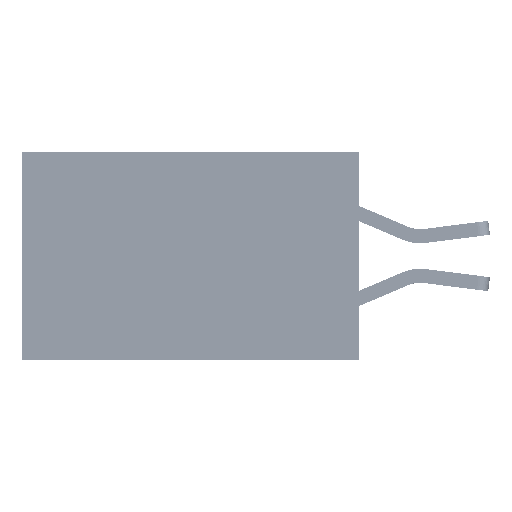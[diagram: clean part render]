
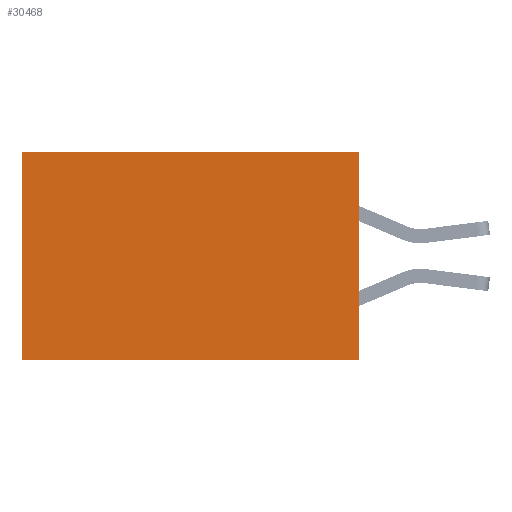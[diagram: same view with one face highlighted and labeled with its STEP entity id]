
A CAD part, left-side view. The second image highlights one B-rep face of the part: STEP entity #30468.
In plain terms, the highlighted planar face has unit normal (-1, 0, 0).
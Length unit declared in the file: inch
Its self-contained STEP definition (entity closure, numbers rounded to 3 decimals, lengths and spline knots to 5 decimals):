
#4207 = LINE ( 'NONE', #34010, #36794 ) ;
#5141 = ORIENTED_EDGE ( 'NONE', *, *, #14940, .T. ) ;
#7392 = VERTEX_POINT ( 'NONE', #22559 ) ;
#9594 = EDGE_LOOP ( 'NONE', ( #5141, #36735, #26626, #35115 ) ) ;
#10495 = PLANE ( 'NONE',  #11909 ) ;
#10801 = CARTESIAN_POINT ( 'NONE',  ( 0.2875, 0., 0. ) ) ;
#11043 = CARTESIAN_POINT ( 'NONE',  ( 0.2875, 0., -0.37 ) ) ;
#11909 = AXIS2_PLACEMENT_3D ( 'NONE', #35470, #16680, #32590 ) ;
#13815 = VERTEX_POINT ( 'NONE', #37390 ) ;
#14940 = EDGE_CURVE ( 'NONE', #33767, #13815, #4207, .T. ) ;
#15058 = DIRECTION ( 'NONE',  ( 0., 0., -1. ) ) ;
#16318 = VECTOR ( 'NONE', #20577, 39.37008 ) ;
#16680 = DIRECTION ( 'NONE',  ( 1., 0., 0. ) ) ;
#19913 = EDGE_CURVE ( 'NONE', #22338, #13815, #20311, .T. ) ;
#20311 = LINE ( 'NONE', #11043, #16318 ) ;
#20577 = DIRECTION ( 'NONE',  ( 0., 1., 0. ) ) ;
#22338 = VERTEX_POINT ( 'NONE', #29741 ) ;
#22379 = VECTOR ( 'NONE', #32746, 39.37008 ) ;
#22559 = CARTESIAN_POINT ( 'NONE',  ( 0.2875, 0., 0. ) ) ;
#22841 = LINE ( 'NONE', #35748, #22379 ) ;
#23680 = FACE_OUTER_BOUND ( 'NONE', #9594, .T. ) ;
#26626 = ORIENTED_EDGE ( 'NONE', *, *, #35046, .F. ) ;
#26760 = VECTOR ( 'NONE', #36186, 39.37008 ) ;
#29741 = CARTESIAN_POINT ( 'NONE',  ( 0.2875, 0., -0.37 ) ) ;
#30468 = ADVANCED_FACE ( 'NONE', ( #23680 ), #10495, .F. ) ;
#32566 = CARTESIAN_POINT ( 'NONE',  ( 0.2875, 0.6, 0. ) ) ;
#32590 = DIRECTION ( 'NONE',  ( 0., 0., -1. ) ) ;
#32746 = DIRECTION ( 'NONE',  ( 0., 0., -1. ) ) ;
#33767 = VERTEX_POINT ( 'NONE', #32566 ) ;
#34010 = CARTESIAN_POINT ( 'NONE',  ( 0.2875, 0.6, 0. ) ) ;
#35046 = EDGE_CURVE ( 'NONE', #7392, #22338, #22841, .T. ) ;
#35115 = ORIENTED_EDGE ( 'NONE', *, *, #40537, .T. ) ;
#35470 = CARTESIAN_POINT ( 'NONE',  ( 0.2875, 0., 0. ) ) ;
#35748 = CARTESIAN_POINT ( 'NONE',  ( 0.2875, 0., 0. ) ) ;
#36186 = DIRECTION ( 'NONE',  ( 0., 1., 0. ) ) ;
#36735 = ORIENTED_EDGE ( 'NONE', *, *, #19913, .F. ) ;
#36794 = VECTOR ( 'NONE', #15058, 39.37008 ) ;
#37390 = CARTESIAN_POINT ( 'NONE',  ( 0.2875, 0.6, -0.37 ) ) ;
#39073 = LINE ( 'NONE', #10801, #26760 ) ;
#40537 = EDGE_CURVE ( 'NONE', #7392, #33767, #39073, .T. ) ;
